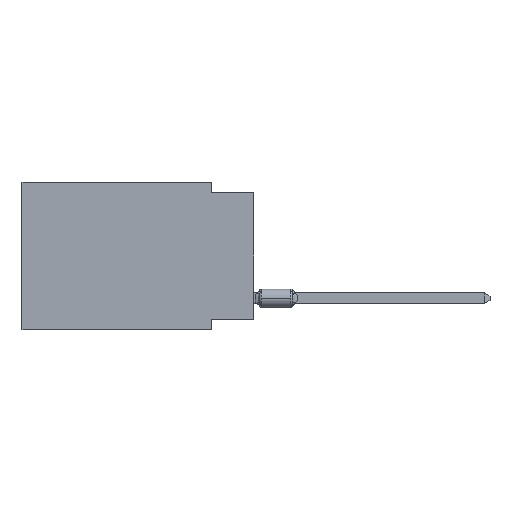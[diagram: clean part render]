
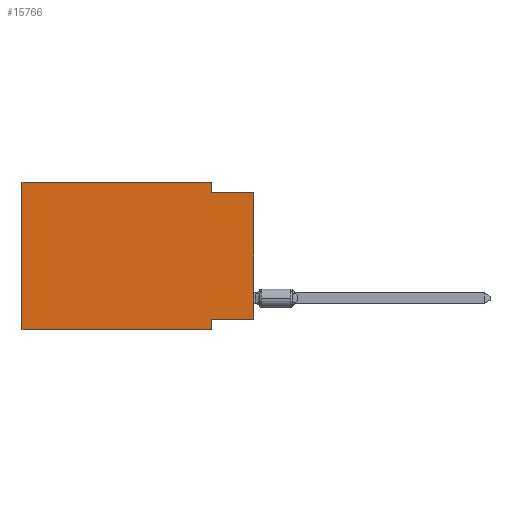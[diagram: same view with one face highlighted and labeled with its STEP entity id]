
A CAD part, left-side view. The second image highlights one B-rep face of the part: STEP entity #15766.
In plain terms, the highlighted planar face has unit normal (-1, 0, 0).
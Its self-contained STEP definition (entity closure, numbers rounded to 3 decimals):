
#103 = ORIENTED_EDGE ( 'NONE', *, *, #2901, .F. ) ;
#586 = CARTESIAN_POINT ( 'NONE',  ( 0., 13.97, 0. ) ) ;
#692 = VECTOR ( 'NONE', #15359, 1000. ) ;
#1553 = DIRECTION ( 'NONE',  ( 0., -1., 0. ) ) ;
#1554 = CARTESIAN_POINT ( 'NONE',  ( 0., 13.97, -8.89 ) ) ;
#2031 = CARTESIAN_POINT ( 'NONE',  ( 0., 13.97, -8.89 ) ) ;
#2217 = VERTEX_POINT ( 'NONE', #14777 ) ;
#2226 = CARTESIAN_POINT ( 'NONE',  ( 0., 2.54, -8.89 ) ) ;
#2593 = EDGE_CURVE ( 'NONE', #14807, #2217, #11264, .T. ) ;
#2708 = ORIENTED_EDGE ( 'NONE', *, *, #5227, .F. ) ;
#2901 = EDGE_CURVE ( 'NONE', #12883, #18013, #10928, .T. ) ;
#3551 = DIRECTION ( 'NONE',  ( 1., 0., 0. ) ) ;
#3843 = VECTOR ( 'NONE', #12506, 1000. ) ;
#4255 = DIRECTION ( 'NONE',  ( 0., 1., 0. ) ) ;
#4525 = VECTOR ( 'NONE', #13425, 1000. ) ;
#4665 = EDGE_CURVE ( 'NONE', #12883, #18255, #19266, .T. ) ;
#4819 = VERTEX_POINT ( 'NONE', #15039 ) ;
#5111 = FACE_OUTER_BOUND ( 'NONE', #17626, .T. ) ;
#5134 = ORIENTED_EDGE ( 'NONE', *, *, #4665, .T. ) ;
#5227 = EDGE_CURVE ( 'NONE', #7998, #14807, #18171, .T. ) ;
#5427 = PLANE ( 'NONE',  #20229 ) ;
#5510 = LINE ( 'NONE', #19968, #8301 ) ;
#5741 = CARTESIAN_POINT ( 'NONE',  ( 0., 0., 0. ) ) ;
#6379 = CARTESIAN_POINT ( 'NONE',  ( 0., 13.97, 0. ) ) ;
#7018 = DIRECTION ( 'NONE',  ( 0., 0., -1. ) ) ;
#7336 = CARTESIAN_POINT ( 'NONE',  ( 0., 2.54, -8.89 ) ) ;
#7514 = EDGE_CURVE ( 'NONE', #4819, #11980, #5510, .T. ) ;
#7823 = CARTESIAN_POINT ( 'NONE',  ( 0., 13.97, 0. ) ) ;
#7898 = EDGE_CURVE ( 'NONE', #11980, #18255, #18470, .T. ) ;
#7998 = VERTEX_POINT ( 'NONE', #13721 ) ;
#8301 = VECTOR ( 'NONE', #4255, 1000. ) ;
#10587 = EDGE_CURVE ( 'NONE', #18013, #7998, #17125, .T. ) ;
#10928 = LINE ( 'NONE', #6379, #3843 ) ;
#11015 = VECTOR ( 'NONE', #20148, 1000. ) ;
#11264 = LINE ( 'NONE', #17591, #20669 ) ;
#11842 = CARTESIAN_POINT ( 'NONE',  ( 0., 2.54, 0. ) ) ;
#11980 = VERTEX_POINT ( 'NONE', #19063 ) ;
#12506 = DIRECTION ( 'NONE',  ( 0., 0., 1. ) ) ;
#12883 = VERTEX_POINT ( 'NONE', #2031 ) ;
#13425 = DIRECTION ( 'NONE',  ( 0., 0., -1. ) ) ;
#13721 = CARTESIAN_POINT ( 'NONE',  ( 0., 2.54, 0. ) ) ;
#13767 = LINE ( 'NONE', #5741, #692 ) ;
#13958 = VECTOR ( 'NONE', #17489, 1000. ) ;
#14330 = ORIENTED_EDGE ( 'NONE', *, *, #2593, .F. ) ;
#14777 = CARTESIAN_POINT ( 'NONE',  ( 0., 0., -0.635 ) ) ;
#14807 = VERTEX_POINT ( 'NONE', #20784 ) ;
#15039 = CARTESIAN_POINT ( 'NONE',  ( 0., 0., -8.255 ) ) ;
#15359 = DIRECTION ( 'NONE',  ( 0., 0., 1. ) ) ;
#15732 = ORIENTED_EDGE ( 'NONE', *, *, #7514, .F. ) ;
#15766 = ADVANCED_FACE ( 'NONE', ( #5111 ), #5427, .F. ) ;
#15924 = EDGE_CURVE ( 'NONE', #4819, #2217, #13767, .T. ) ;
#17125 = LINE ( 'NONE', #7823, #20795 ) ;
#17192 = CARTESIAN_POINT ( 'NONE',  ( 0., 13.97, 0. ) ) ;
#17489 = DIRECTION ( 'NONE',  ( 0., -1., 0. ) ) ;
#17591 = CARTESIAN_POINT ( 'NONE',  ( 0., 0., -0.635 ) ) ;
#17626 = EDGE_LOOP ( 'NONE', ( #19804, #14330, #2708, #17780, #103, #5134, #20113, #15732 ) ) ;
#17780 = ORIENTED_EDGE ( 'NONE', *, *, #10587, .F. ) ;
#18013 = VERTEX_POINT ( 'NONE', #17192 ) ;
#18171 = LINE ( 'NONE', #11842, #4525 ) ;
#18255 = VERTEX_POINT ( 'NONE', #7336 ) ;
#18470 = LINE ( 'NONE', #2226, #11015 ) ;
#19063 = CARTESIAN_POINT ( 'NONE',  ( 0., 2.54, -8.255 ) ) ;
#19266 = LINE ( 'NONE', #1554, #13958 ) ;
#19804 = ORIENTED_EDGE ( 'NONE', *, *, #15924, .T. ) ;
#19968 = CARTESIAN_POINT ( 'NONE',  ( 0., 0., -8.255 ) ) ;
#20113 = ORIENTED_EDGE ( 'NONE', *, *, #7898, .F. ) ;
#20148 = DIRECTION ( 'NONE',  ( 0., 0., -1. ) ) ;
#20181 = DIRECTION ( 'NONE',  ( 0., -1., 0. ) ) ;
#20229 = AXIS2_PLACEMENT_3D ( 'NONE', #586, #3551, #7018 ) ;
#20669 = VECTOR ( 'NONE', #1553, 1000. ) ;
#20784 = CARTESIAN_POINT ( 'NONE',  ( 0., 2.54, -0.635 ) ) ;
#20795 = VECTOR ( 'NONE', #20181, 1000. ) ;
